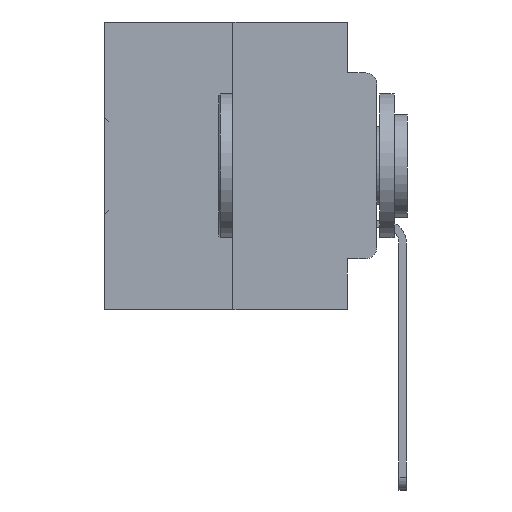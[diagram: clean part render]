
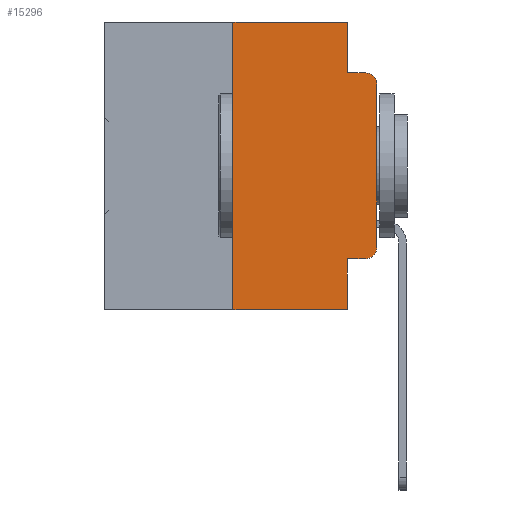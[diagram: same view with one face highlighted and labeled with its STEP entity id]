
A CAD part, left-side view. The second image highlights one B-rep face of the part: STEP entity #15296.
In plain terms, the highlighted planar face has unit normal (-1, 0, 0).
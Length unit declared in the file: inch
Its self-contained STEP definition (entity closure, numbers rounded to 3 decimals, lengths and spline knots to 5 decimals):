
#793 = VERTEX_POINT ( 'NONE', #31184 ) ;
#975 = LINE ( 'NONE', #3884, #12925 ) ;
#1307 = CARTESIAN_POINT ( 'NONE',  ( 0., 0.25, 0. ) ) ;
#1369 = EDGE_CURVE ( 'NONE', #26702, #22826, #27512, .T. ) ;
#1396 = ORIENTED_EDGE ( 'NONE', *, *, #28449, .T. ) ;
#1422 = VECTOR ( 'NONE', #28504, 39.37008 ) ;
#1453 = VERTEX_POINT ( 'NONE', #26244 ) ;
#1678 = EDGE_LOOP ( 'NONE', ( #1396, #15813, #23882, #19478, #28420, #2151, #16518, #24627, #11124, #25472 ) ) ;
#1995 = DIRECTION ( 'NONE',  ( 0., -1., 0. ) ) ;
#2151 = ORIENTED_EDGE ( 'NONE', *, *, #15709, .F. ) ;
#2284 = LINE ( 'NONE', #13843, #34689 ) ;
#2538 = DIRECTION ( 'NONE',  ( 0., 0., -1. ) ) ;
#3480 = VECTOR ( 'NONE', #27044, 39.37008 ) ;
#3884 = CARTESIAN_POINT ( 'NONE',  ( 0., 0., 0. ) ) ;
#4153 = EDGE_CURVE ( 'NONE', #1453, #7565, #7891, .T. ) ;
#4905 = EDGE_CURVE ( 'NONE', #6750, #16994, #26394, .T. ) ;
#5451 = PLANE ( 'NONE',  #30575 ) ;
#6746 = EDGE_CURVE ( 'NONE', #10788, #6750, #31326, .T. ) ;
#6750 = VERTEX_POINT ( 'NONE', #21570 ) ;
#6916 = CARTESIAN_POINT ( 'NONE',  ( 0., 0.473, 0. ) ) ;
#7537 = CARTESIAN_POINT ( 'NONE',  ( 0., 0.051, -0.0885 ) ) ;
#7565 = VERTEX_POINT ( 'NONE', #27708 ) ;
#7685 = VERTEX_POINT ( 'NONE', #21439 ) ;
#7891 = LINE ( 'NONE', #25781, #1422 ) ;
#8162 = CARTESIAN_POINT ( 'NONE',  ( 0., 0.051, -0.4115 ) ) ;
#8395 = CARTESIAN_POINT ( 'NONE',  ( 0., 0.051, -0.4115 ) ) ;
#9202 = LINE ( 'NONE', #10021, #28212 ) ;
#10021 = CARTESIAN_POINT ( 'NONE',  ( 0., 0.25, 0. ) ) ;
#10775 = LINE ( 'NONE', #7537, #17021 ) ;
#10788 = VERTEX_POINT ( 'NONE', #8395 ) ;
#11124 = ORIENTED_EDGE ( 'NONE', *, *, #6746, .T. ) ;
#11389 = DIRECTION ( 'NONE',  ( 0., 0., -1. ) ) ;
#11966 = DIRECTION ( 'NONE',  ( 0., 0., 1. ) ) ;
#12166 = EDGE_CURVE ( 'NONE', #10788, #7565, #25855, .T. ) ;
#12340 = VECTOR ( 'NONE', #11389, 39.37008 ) ;
#12925 = VECTOR ( 'NONE', #11966, 39.37008 ) ;
#13118 = VECTOR ( 'NONE', #23163, 39.37008 ) ;
#13557 = DIRECTION ( 'NONE',  ( 1., 0., 0. ) ) ;
#13843 = CARTESIAN_POINT ( 'NONE',  ( 0., 0.051, 0. ) ) ;
#14727 = CARTESIAN_POINT ( 'NONE',  ( 0., 0.02, -0.1085 ) ) ;
#15296 = ADVANCED_FACE ( 'NONE', ( #29071 ), #5451, .F. ) ;
#15557 = CARTESIAN_POINT ( 'NONE',  ( 0., 0.051, 0. ) ) ;
#15709 = EDGE_CURVE ( 'NONE', #1453, #26702, #9202, .T. ) ;
#15813 = ORIENTED_EDGE ( 'NONE', *, *, #26630, .T. ) ;
#16500 = DIRECTION ( 'NONE',  ( 0., 0., -1. ) ) ;
#16518 = ORIENTED_EDGE ( 'NONE', *, *, #4153, .T. ) ;
#16994 = VERTEX_POINT ( 'NONE', #24759 ) ;
#17021 = VECTOR ( 'NONE', #1995, 39.37008 ) ;
#17426 = DIRECTION ( 'NONE',  ( 0., 0., -1. ) ) ;
#17528 = EDGE_CURVE ( 'NONE', #22826, #7685, #2284, .T. ) ;
#18717 = DIRECTION ( 'NONE',  ( -1., 0., 0. ) ) ;
#19478 = ORIENTED_EDGE ( 'NONE', *, *, #17528, .F. ) ;
#21147 = EDGE_CURVE ( 'NONE', #7685, #28987, #10775, .T. ) ;
#21439 = CARTESIAN_POINT ( 'NONE',  ( 0., 0.051, -0.0885 ) ) ;
#21570 = CARTESIAN_POINT ( 'NONE',  ( 0., 0.02, -0.4115 ) ) ;
#21577 = CARTESIAN_POINT ( 'NONE',  ( 0., 0.473, 0. ) ) ;
#22826 = VERTEX_POINT ( 'NONE', #15557 ) ;
#23163 = DIRECTION ( 'NONE',  ( 0., -1., 0. ) ) ;
#23882 = ORIENTED_EDGE ( 'NONE', *, *, #21147, .F. ) ;
#24627 = ORIENTED_EDGE ( 'NONE', *, *, #12166, .F. ) ;
#24759 = CARTESIAN_POINT ( 'NONE',  ( 0., 0., -0.3915 ) ) ;
#24850 = CARTESIAN_POINT ( 'NONE',  ( 0., 0.051, 0. ) ) ;
#25472 = ORIENTED_EDGE ( 'NONE', *, *, #4905, .T. ) ;
#25781 = CARTESIAN_POINT ( 'NONE',  ( 0., 0.473, -0.5 ) ) ;
#25855 = LINE ( 'NONE', #24850, #12340 ) ;
#26244 = CARTESIAN_POINT ( 'NONE',  ( 0., 0.25, -0.5 ) ) ;
#26360 = AXIS2_PLACEMENT_3D ( 'NONE', #14727, #33504, #17426 ) ;
#26394 = CIRCLE ( 'NONE', #28328, 0.02 ) ;
#26630 = EDGE_CURVE ( 'NONE', #793, #28987, #27444, .T. ) ;
#26702 = VERTEX_POINT ( 'NONE', #1307 ) ;
#27044 = DIRECTION ( 'NONE',  ( 0., -1., 0. ) ) ;
#27444 = CIRCLE ( 'NONE', #26360, 0.02 ) ;
#27512 = LINE ( 'NONE', #6916, #13118 ) ;
#27708 = CARTESIAN_POINT ( 'NONE',  ( 0., 0.051, -0.5 ) ) ;
#28212 = VECTOR ( 'NONE', #34142, 39.37008 ) ;
#28328 = AXIS2_PLACEMENT_3D ( 'NONE', #34758, #18717, #2538 ) ;
#28420 = ORIENTED_EDGE ( 'NONE', *, *, #1369, .F. ) ;
#28449 = EDGE_CURVE ( 'NONE', #16994, #793, #975, .T. ) ;
#28504 = DIRECTION ( 'NONE',  ( 0., -1., 0. ) ) ;
#28987 = VERTEX_POINT ( 'NONE', #30645 ) ;
#29071 = FACE_OUTER_BOUND ( 'NONE', #1678, .T. ) ;
#30575 = AXIS2_PLACEMENT_3D ( 'NONE', #21577, #13557, #32381 ) ;
#30645 = CARTESIAN_POINT ( 'NONE',  ( 0., 0.02, -0.0885 ) ) ;
#31184 = CARTESIAN_POINT ( 'NONE',  ( 0., 0., -0.1085 ) ) ;
#31326 = LINE ( 'NONE', #8162, #3480 ) ;
#32381 = DIRECTION ( 'NONE',  ( 0., 0., -1. ) ) ;
#33504 = DIRECTION ( 'NONE',  ( -1., 0., 0. ) ) ;
#34142 = DIRECTION ( 'NONE',  ( 0., 0., 1. ) ) ;
#34689 = VECTOR ( 'NONE', #16500, 39.37008 ) ;
#34758 = CARTESIAN_POINT ( 'NONE',  ( 0., 0.02, -0.3915 ) ) ;
